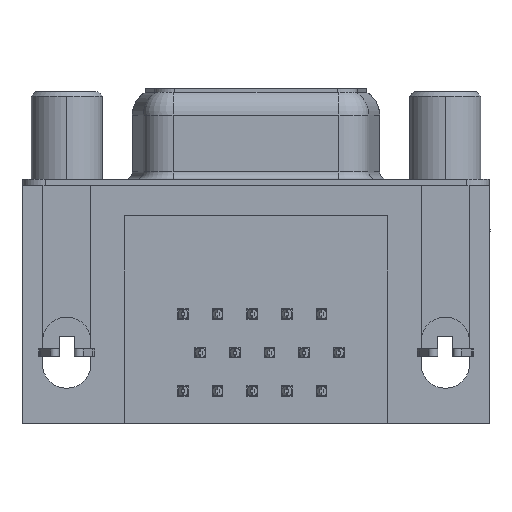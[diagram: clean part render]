
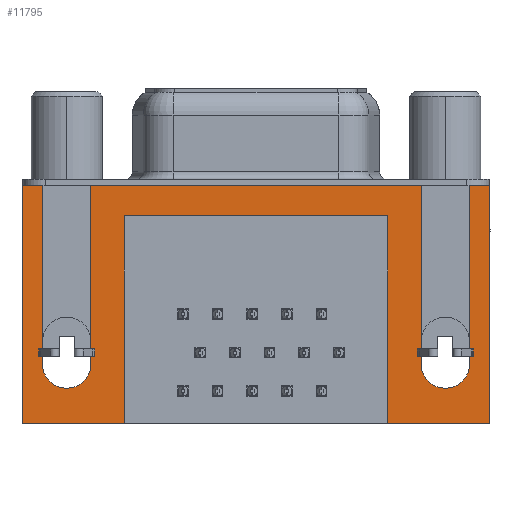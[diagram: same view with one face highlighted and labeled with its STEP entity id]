
A CAD part, front view. The second image highlights one B-rep face of the part: STEP entity #11795.
In plain terms, the highlighted planar face has unit normal (0, -1, 0).
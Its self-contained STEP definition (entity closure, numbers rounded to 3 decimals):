
#112 = EDGE_CURVE ( 'NONE', #1625, #26037, #5915, .T. ) ;
#309 = CARTESIAN_POINT ( 'NONE',  ( 3.79, -6.275, -15.7 ) ) ;
#424 = DIRECTION ( 'NONE',  ( 0., 0., 1. ) ) ;
#520 = EDGE_CURVE ( 'NONE', #23369, #35727, #36639, .T. ) ;
#561 = CARTESIAN_POINT ( 'NONE',  ( 21.2, -6.275, -15.7 ) ) ;
#840 = CARTESIAN_POINT ( 'NONE',  ( 1.6, -6.275, 0. ) ) ;
#1170 = DIRECTION ( 'NONE',  ( -1., 0., 0. ) ) ;
#1286 = VERTEX_POINT ( 'NONE', #34564 ) ;
#1605 = ORIENTED_EDGE ( 'NONE', *, *, #29559, .F. ) ;
#1625 = VERTEX_POINT ( 'NONE', #24872 ) ;
#2653 = ORIENTED_EDGE ( 'NONE', *, *, #30117, .F. ) ;
#3421 = DIRECTION ( 'NONE',  ( 0., 0., -1. ) ) ;
#3664 = PLANE ( 'NONE',  #18721 ) ;
#3941 = DIRECTION ( 'NONE',  ( 0., -1., 0. ) ) ;
#4085 = CARTESIAN_POINT ( 'NONE',  ( -2.91, -6.275, 0. ) ) ;
#4342 = CARTESIAN_POINT ( 'NONE',  ( -2.91, -6.275, 0. ) ) ;
#4484 = CARTESIAN_POINT ( 'NONE',  ( -2.91, -6.275, -2.5 ) ) ;
#4843 = DIRECTION ( 'NONE',  ( 0., 0., 1. ) ) ;
#5074 = VECTOR ( 'NONE', #32541, 1000. ) ;
#5256 = LINE ( 'NONE', #4085, #25077 ) ;
#5427 = VECTOR ( 'NONE', #1170, 1000. ) ;
#5649 = DIRECTION ( 'NONE',  ( 0., 0., -1. ) ) ;
#5672 = CARTESIAN_POINT ( 'NONE',  ( 1.6, -6.275, -11.78 ) ) ;
#5774 = LINE ( 'NONE', #24080, #25581 ) ;
#5915 = LINE ( 'NONE', #4484, #35282 ) ;
#6031 = VERTEX_POINT ( 'NONE', #36684 ) ;
#6795 = CARTESIAN_POINT ( 'NONE',  ( 27.9, -6.275, -2.5 ) ) ;
#7910 = EDGE_CURVE ( 'NONE', #23369, #19874, #31081, .T. ) ;
#8043 = VERTEX_POINT ( 'NONE', #24670 ) ;
#8614 = VECTOR ( 'NONE', #27351, 1000. ) ;
#8845 = EDGE_CURVE ( 'NONE', #37605, #6031, #5774, .T. ) ;
#8998 = CARTESIAN_POINT ( 'NONE',  ( 27.9, -6.275, -15.7 ) ) ;
#9395 = VERTEX_POINT ( 'NONE', #37479 ) ;
#9463 = DIRECTION ( 'NONE',  ( 0., 0., 1. ) ) ;
#9679 = CARTESIAN_POINT ( 'NONE',  ( -2.91, -6.275, -2.5 ) ) ;
#9999 = VERTEX_POINT ( 'NONE', #36945 ) ;
#10351 = EDGE_LOOP ( 'NONE', ( #26595, #29203, #17104, #29172, #25471, #1605, #24365, #27475, #29263, #19062, #15870, #23104, #17606, #34771, #21014, #2653 ) ) ;
#10720 = CARTESIAN_POINT ( 'NONE',  ( -1.6, -6.275, 0. ) ) ;
#10896 = CARTESIAN_POINT ( 'NONE',  ( 27.9, -6.275, 0. ) ) ;
#11018 = DIRECTION ( 'NONE',  ( -1., 0., 0. ) ) ;
#11524 = VECTOR ( 'NONE', #36063, 1000. ) ;
#11795 = ADVANCED_FACE ( 'NONE', ( #33491 ), #3664, .T. ) ;
#11952 = CARTESIAN_POINT ( 'NONE',  ( 24.99, -6.275, -11.78 ) ) ;
#12397 = CARTESIAN_POINT ( 'NONE',  ( 3.79, -6.275, -2. ) ) ;
#12679 = DIRECTION ( 'NONE',  ( 0., 0., -1. ) ) ;
#13444 = VECTOR ( 'NONE', #31151, 1000. ) ;
#14335 = VECTOR ( 'NONE', #24955, 1000. ) ;
#14932 = DIRECTION ( 'NONE',  ( -1., 0., 0. ) ) ;
#15420 = VERTEX_POINT ( 'NONE', #36086 ) ;
#15870 = ORIENTED_EDGE ( 'NONE', *, *, #34178, .F. ) ;
#16624 = CARTESIAN_POINT ( 'NONE',  ( 26.59, -6.275, -11.78 ) ) ;
#17104 = ORIENTED_EDGE ( 'NONE', *, *, #34324, .F. ) ;
#17297 = VERTEX_POINT ( 'NONE', #32832 ) ;
#17606 = ORIENTED_EDGE ( 'NONE', *, *, #33277, .F. ) ;
#17757 = VECTOR ( 'NONE', #11018, 1000. ) ;
#18691 = LINE ( 'NONE', #28514, #17757 ) ;
#18698 = AXIS2_PLACEMENT_3D ( 'NONE', #11952, #32367, #14932 ) ;
#18721 = AXIS2_PLACEMENT_3D ( 'NONE', #9679, #30139, #12679 ) ;
#18731 = VECTOR ( 'NONE', #27320, 1000. ) ;
#18894 = EDGE_CURVE ( 'NONE', #1286, #15420, #5256, .T. ) ;
#19062 = ORIENTED_EDGE ( 'NONE', *, *, #30703, .F. ) ;
#19829 = LINE ( 'NONE', #26873, #26686 ) ;
#19874 = VERTEX_POINT ( 'NONE', #10896 ) ;
#20038 = VERTEX_POINT ( 'NONE', #309 ) ;
#20273 = LINE ( 'NONE', #10720, #13444 ) ;
#21014 = ORIENTED_EDGE ( 'NONE', *, *, #7910, .T. ) ;
#21140 = CARTESIAN_POINT ( 'NONE',  ( 21.2, -6.275, -2. ) ) ;
#21554 = CIRCLE ( 'NONE', #18698, 1.6 ) ;
#21655 = CARTESIAN_POINT ( 'NONE',  ( 0., -6.275, -11.78 ) ) ;
#22738 = EDGE_CURVE ( 'NONE', #17297, #9999, #20273, .T. ) ;
#22854 = CIRCLE ( 'NONE', #31290, 1.6 ) ;
#23104 = ORIENTED_EDGE ( 'NONE', *, *, #33735, .F. ) ;
#23369 = VERTEX_POINT ( 'NONE', #32867 ) ;
#23375 = EDGE_CURVE ( 'NONE', #25666, #1286, #27095, .T. ) ;
#23488 = LINE ( 'NONE', #26242, #38031 ) ;
#23994 = LINE ( 'NONE', #21140, #31728 ) ;
#24080 = CARTESIAN_POINT ( 'NONE',  ( 26.59, -6.275, 0. ) ) ;
#24365 = ORIENTED_EDGE ( 'NONE', *, *, #22738, .F. ) ;
#24563 = DIRECTION ( 'NONE',  ( 1., 0., 0. ) ) ;
#24670 = CARTESIAN_POINT ( 'NONE',  ( 23.39, -6.275, -11.78 ) ) ;
#24872 = CARTESIAN_POINT ( 'NONE',  ( -2.91, -6.275, -15.7 ) ) ;
#24955 = DIRECTION ( 'NONE',  ( 1., 0., 0. ) ) ;
#25077 = VECTOR ( 'NONE', #33489, 1000. ) ;
#25471 = ORIENTED_EDGE ( 'NONE', *, *, #23375, .F. ) ;
#25548 = CARTESIAN_POINT ( 'NONE',  ( 3.79, -6.275, -2. ) ) ;
#25581 = VECTOR ( 'NONE', #9463, 1000. ) ;
#25666 = VERTEX_POINT ( 'NONE', #5672 ) ;
#26037 = VERTEX_POINT ( 'NONE', #35629 ) ;
#26242 = CARTESIAN_POINT ( 'NONE',  ( 3.79, -6.275, -2. ) ) ;
#26455 = LINE ( 'NONE', #30245, #18731 ) ;
#26595 = ORIENTED_EDGE ( 'NONE', *, *, #8845, .F. ) ;
#26686 = VECTOR ( 'NONE', #3421, 1000. ) ;
#26873 = CARTESIAN_POINT ( 'NONE',  ( 23.39, -6.275, 0. ) ) ;
#27095 = LINE ( 'NONE', #840, #11524 ) ;
#27320 = DIRECTION ( 'NONE',  ( 1., 0., 0. ) ) ;
#27351 = DIRECTION ( 'NONE',  ( 0., 0., 1. ) ) ;
#27475 = ORIENTED_EDGE ( 'NONE', *, *, #34486, .F. ) ;
#27618 = LINE ( 'NONE', #12397, #5074 ) ;
#28514 = CARTESIAN_POINT ( 'NONE',  ( 27.9, -6.275, -15.7 ) ) ;
#29172 = ORIENTED_EDGE ( 'NONE', *, *, #18894, .F. ) ;
#29203 = ORIENTED_EDGE ( 'NONE', *, *, #37780, .F. ) ;
#29263 = ORIENTED_EDGE ( 'NONE', *, *, #112, .F. ) ;
#29559 = EDGE_CURVE ( 'NONE', #9999, #25666, #22854, .T. ) ;
#30117 = EDGE_CURVE ( 'NONE', #6031, #19874, #26455, .T. ) ;
#30139 = DIRECTION ( 'NONE',  ( 0., -1., 0. ) ) ;
#30245 = CARTESIAN_POINT ( 'NONE',  ( -2.91, -6.275, 0. ) ) ;
#30703 = EDGE_CURVE ( 'NONE', #20038, #1625, #18691, .T. ) ;
#31081 = LINE ( 'NONE', #6795, #8614 ) ;
#31151 = DIRECTION ( 'NONE',  ( 0., 0., -1. ) ) ;
#31290 = AXIS2_PLACEMENT_3D ( 'NONE', #21655, #3941, #24563 ) ;
#31728 = VECTOR ( 'NONE', #424, 1000. ) ;
#32367 = DIRECTION ( 'NONE',  ( 0., -1., 0. ) ) ;
#32541 = DIRECTION ( 'NONE',  ( -1., 0., 0. ) ) ;
#32832 = CARTESIAN_POINT ( 'NONE',  ( -1.6, -6.275, 0. ) ) ;
#32867 = CARTESIAN_POINT ( 'NONE',  ( 27.9, -6.275, -15.7 ) ) ;
#33277 = EDGE_CURVE ( 'NONE', #35727, #9395, #23994, .T. ) ;
#33489 = DIRECTION ( 'NONE',  ( 1., 0., 0. ) ) ;
#33491 = FACE_OUTER_BOUND ( 'NONE', #10351, .T. ) ;
#33735 = EDGE_CURVE ( 'NONE', #9395, #35029, #27618, .T. ) ;
#34178 = EDGE_CURVE ( 'NONE', #35029, #20038, #23488, .T. ) ;
#34324 = EDGE_CURVE ( 'NONE', #15420, #8043, #19829, .T. ) ;
#34486 = EDGE_CURVE ( 'NONE', #26037, #17297, #36690, .T. ) ;
#34564 = CARTESIAN_POINT ( 'NONE',  ( 1.6, -6.275, 0. ) ) ;
#34771 = ORIENTED_EDGE ( 'NONE', *, *, #520, .F. ) ;
#35029 = VERTEX_POINT ( 'NONE', #25548 ) ;
#35282 = VECTOR ( 'NONE', #4843, 1000. ) ;
#35629 = CARTESIAN_POINT ( 'NONE',  ( -2.91, -6.275, 0. ) ) ;
#35727 = VERTEX_POINT ( 'NONE', #561 ) ;
#36063 = DIRECTION ( 'NONE',  ( 0., 0., 1. ) ) ;
#36086 = CARTESIAN_POINT ( 'NONE',  ( 23.39, -6.275, 0. ) ) ;
#36639 = LINE ( 'NONE', #8998, #5427 ) ;
#36684 = CARTESIAN_POINT ( 'NONE',  ( 26.59, -6.275, 0. ) ) ;
#36690 = LINE ( 'NONE', #4342, #14335 ) ;
#36945 = CARTESIAN_POINT ( 'NONE',  ( -1.6, -6.275, -11.78 ) ) ;
#37479 = CARTESIAN_POINT ( 'NONE',  ( 21.2, -6.275, -2. ) ) ;
#37605 = VERTEX_POINT ( 'NONE', #16624 ) ;
#37780 = EDGE_CURVE ( 'NONE', #8043, #37605, #21554, .T. ) ;
#38031 = VECTOR ( 'NONE', #5649, 1000. ) ;
